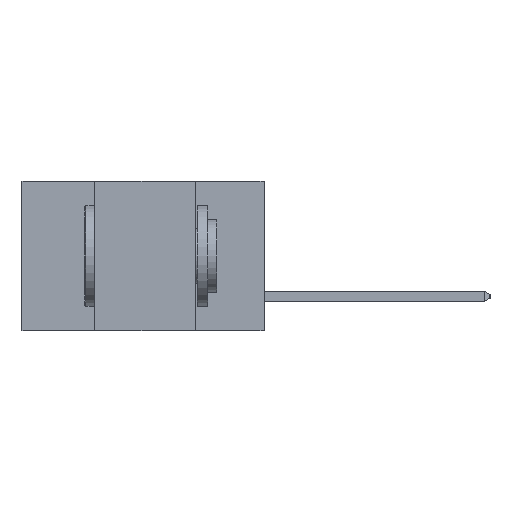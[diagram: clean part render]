
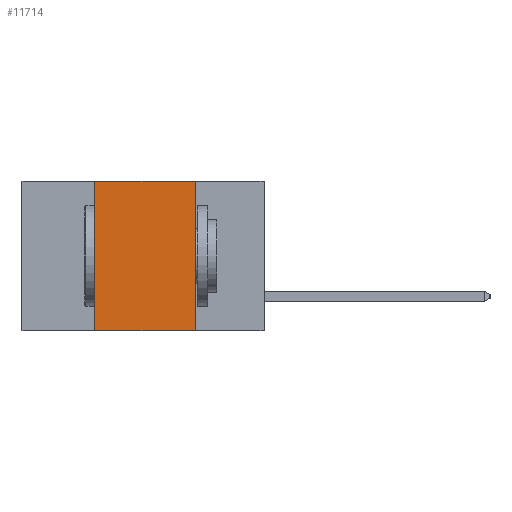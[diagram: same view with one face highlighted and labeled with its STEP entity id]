
A CAD part, left-side view. The second image highlights one B-rep face of the part: STEP entity #11714.
In plain terms, the highlighted planar face has unit normal (-1, 0, 0).
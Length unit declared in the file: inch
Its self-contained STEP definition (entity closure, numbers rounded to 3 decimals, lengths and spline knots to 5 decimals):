
#89 = ORIENTED_EDGE ( 'NONE', *, *, #15411, .F. ) ;
#421 = VECTOR ( 'NONE', #15649, 39.37008 ) ;
#613 = EDGE_LOOP ( 'NONE', ( #6715, #18249, #89, #19929 ) ) ;
#1494 = LINE ( 'NONE', #20645, #421 ) ;
#1569 = CARTESIAN_POINT ( 'NONE',  ( 0., 0.42, -0.37 ) ) ;
#2607 = CARTESIAN_POINT ( 'NONE',  ( 0., 0.42, -0.37 ) ) ;
#2929 = LINE ( 'NONE', #2607, #6641 ) ;
#4297 = DIRECTION ( 'NONE',  ( 0., 0., 1. ) ) ;
#4406 = FACE_OUTER_BOUND ( 'NONE', #613, .T. ) ;
#4428 = VECTOR ( 'NONE', #11694, 39.37008 ) ;
#4907 = VERTEX_POINT ( 'NONE', #18242 ) ;
#6641 = VECTOR ( 'NONE', #4297, 39.37008 ) ;
#6715 = ORIENTED_EDGE ( 'NONE', *, *, #14163, .F. ) ;
#7052 = VERTEX_POINT ( 'NONE', #18595 ) ;
#9866 = VECTOR ( 'NONE', #18814, 39.37008 ) ;
#11284 = EDGE_CURVE ( 'NONE', #15634, #7052, #17818, .T. ) ;
#11694 = DIRECTION ( 'NONE',  ( 0., -1., 0. ) ) ;
#11714 = ADVANCED_FACE ( 'NONE', ( #4406 ), #21393, .F. ) ;
#11746 = CARTESIAN_POINT ( 'NONE',  ( 0., 0.6, -0.37 ) ) ;
#12057 = AXIS2_PLACEMENT_3D ( 'NONE', #21234, #20799, #20796 ) ;
#13769 = EDGE_CURVE ( 'NONE', #4907, #20858, #1494, .T. ) ;
#14163 = EDGE_CURVE ( 'NONE', #20858, #7052, #19232, .T. ) ;
#15411 = EDGE_CURVE ( 'NONE', #15634, #4907, #2929, .T. ) ;
#15634 = VERTEX_POINT ( 'NONE', #1569 ) ;
#15649 = DIRECTION ( 'NONE',  ( 0., -1., 0. ) ) ;
#16280 = CARTESIAN_POINT ( 'NONE',  ( 0., 0.17, 0. ) ) ;
#17818 = LINE ( 'NONE', #11746, #4428 ) ;
#18242 = CARTESIAN_POINT ( 'NONE',  ( 0., 0.42, 0. ) ) ;
#18249 = ORIENTED_EDGE ( 'NONE', *, *, #13769, .F. ) ;
#18595 = CARTESIAN_POINT ( 'NONE',  ( 0., 0.17, -0.37 ) ) ;
#18814 = DIRECTION ( 'NONE',  ( 0., 0., -1. ) ) ;
#19232 = LINE ( 'NONE', #19669, #9866 ) ;
#19669 = CARTESIAN_POINT ( 'NONE',  ( 0., 0.17, -0.37 ) ) ;
#19929 = ORIENTED_EDGE ( 'NONE', *, *, #11284, .T. ) ;
#20645 = CARTESIAN_POINT ( 'NONE',  ( 0., 0.6, 0. ) ) ;
#20796 = DIRECTION ( 'NONE',  ( 0., 0., -1. ) ) ;
#20799 = DIRECTION ( 'NONE',  ( 1., 0., 0. ) ) ;
#20858 = VERTEX_POINT ( 'NONE', #16280 ) ;
#21234 = CARTESIAN_POINT ( 'NONE',  ( 0., 0.6, 0. ) ) ;
#21393 = PLANE ( 'NONE',  #12057 ) ;
